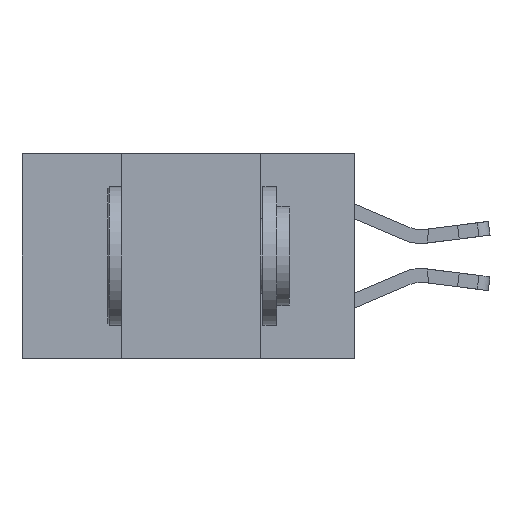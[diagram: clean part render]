
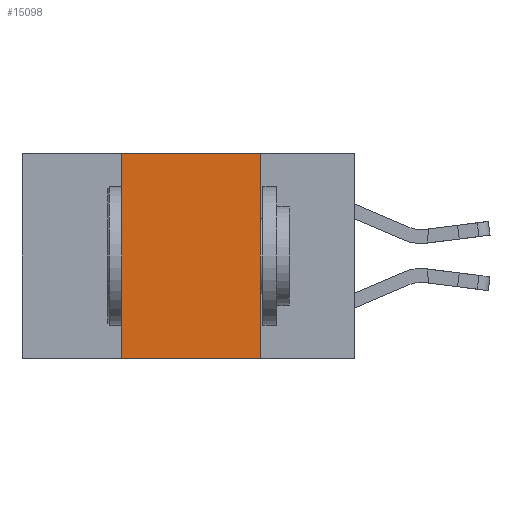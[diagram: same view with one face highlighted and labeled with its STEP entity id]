
A CAD part, left-side view. The second image highlights one B-rep face of the part: STEP entity #15098.
In plain terms, the highlighted planar face has unit normal (-1, 0, 0).
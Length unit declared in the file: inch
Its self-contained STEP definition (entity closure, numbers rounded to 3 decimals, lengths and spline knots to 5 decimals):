
#1690 = EDGE_LOOP ( 'NONE', ( #11105, #11685, #12256, #19204 ) ) ;
#1711 = EDGE_CURVE ( 'NONE', #16599, #11926, #12936, .T. ) ;
#2074 = LINE ( 'NONE', #16458, #20715 ) ;
#2313 = PLANE ( 'NONE',  #5980 ) ;
#3366 = CARTESIAN_POINT ( 'NONE',  ( 0., 0.17, -0.37 ) ) ;
#3404 = VECTOR ( 'NONE', #8174, 39.37008 ) ;
#4178 = DIRECTION ( 'NONE',  ( 1., 0., 0. ) ) ;
#5072 = VERTEX_POINT ( 'NONE', #9483 ) ;
#5980 = AXIS2_PLACEMENT_3D ( 'NONE', #15077, #4178, #16832 ) ;
#6076 = EDGE_CURVE ( 'NONE', #5072, #11926, #7461, .T. ) ;
#7007 = VERTEX_POINT ( 'NONE', #14735 ) ;
#7461 = LINE ( 'NONE', #20169, #8036 ) ;
#8036 = VECTOR ( 'NONE', #20304, 39.37008 ) ;
#8174 = DIRECTION ( 'NONE',  ( 0., -1., 0. ) ) ;
#8945 = CARTESIAN_POINT ( 'NONE',  ( 0., 0.6, -0.37 ) ) ;
#9259 = DIRECTION ( 'NONE',  ( 0., 0., 1. ) ) ;
#9483 = CARTESIAN_POINT ( 'NONE',  ( 0., 0.17, 0. ) ) ;
#11105 = ORIENTED_EDGE ( 'NONE', *, *, #6076, .F. ) ;
#11685 = ORIENTED_EDGE ( 'NONE', *, *, #14580, .F. ) ;
#11926 = VERTEX_POINT ( 'NONE', #3366 ) ;
#12256 = ORIENTED_EDGE ( 'NONE', *, *, #17435, .F. ) ;
#12369 = VECTOR ( 'NONE', #19341, 39.37008 ) ;
#12936 = LINE ( 'NONE', #8945, #12369 ) ;
#14580 = EDGE_CURVE ( 'NONE', #7007, #5072, #21932, .T. ) ;
#14735 = CARTESIAN_POINT ( 'NONE',  ( 0., 0.42, 0. ) ) ;
#15077 = CARTESIAN_POINT ( 'NONE',  ( 0., 0.6, 0. ) ) ;
#15098 = ADVANCED_FACE ( 'NONE', ( #16146 ), #2313, .F. ) ;
#16146 = FACE_OUTER_BOUND ( 'NONE', #1690, .T. ) ;
#16458 = CARTESIAN_POINT ( 'NONE',  ( 0., 0.42, 0. ) ) ;
#16599 = VERTEX_POINT ( 'NONE', #21244 ) ;
#16832 = DIRECTION ( 'NONE',  ( 0., 0., -1. ) ) ;
#17435 = EDGE_CURVE ( 'NONE', #16599, #7007, #2074, .T. ) ;
#19004 = CARTESIAN_POINT ( 'NONE',  ( 0., 0.6, 0. ) ) ;
#19204 = ORIENTED_EDGE ( 'NONE', *, *, #1711, .T. ) ;
#19341 = DIRECTION ( 'NONE',  ( 0., -1., 0. ) ) ;
#20169 = CARTESIAN_POINT ( 'NONE',  ( 0., 0.17, 0. ) ) ;
#20304 = DIRECTION ( 'NONE',  ( 0., 0., -1. ) ) ;
#20715 = VECTOR ( 'NONE', #9259, 39.37008 ) ;
#21244 = CARTESIAN_POINT ( 'NONE',  ( 0., 0.42, -0.37 ) ) ;
#21932 = LINE ( 'NONE', #19004, #3404 ) ;
